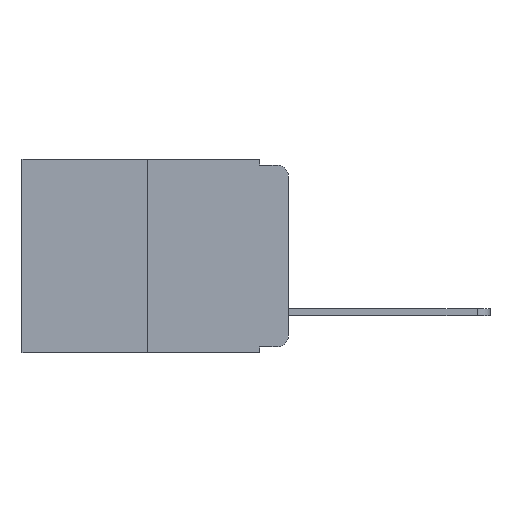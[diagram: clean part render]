
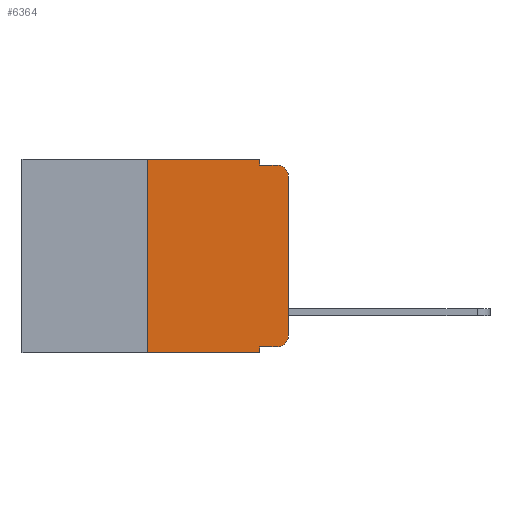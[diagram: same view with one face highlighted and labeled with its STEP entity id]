
A CAD part, left-side view. The second image highlights one B-rep face of the part: STEP entity #6364.
In plain terms, the highlighted planar face has unit normal (-1, 0, 0).
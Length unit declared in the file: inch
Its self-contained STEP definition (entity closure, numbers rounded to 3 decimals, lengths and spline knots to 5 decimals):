
#136 = CARTESIAN_POINT ( 'NONE',  ( 0., 0.02, -0.01 ) ) ;
#164 = CARTESIAN_POINT ( 'NONE',  ( 0., 0.051, 0. ) ) ;
#238 = EDGE_CURVE ( 'NONE', #1976, #2166, #1881, .T. ) ;
#375 = PLANE ( 'NONE',  #6137 ) ;
#435 = CARTESIAN_POINT ( 'NONE',  ( 0., 0.25, -0.343 ) ) ;
#563 = ORIENTED_EDGE ( 'NONE', *, *, #2200, .T. ) ;
#633 = VERTEX_POINT ( 'NONE', #4123 ) ;
#638 = FACE_OUTER_BOUND ( 'NONE', #3313, .T. ) ;
#803 = ORIENTED_EDGE ( 'NONE', *, *, #2149, .F. ) ;
#841 = VERTEX_POINT ( 'NONE', #3508 ) ;
#1305 = VERTEX_POINT ( 'NONE', #435 ) ;
#1477 = DIRECTION ( 'NONE',  ( 1., 0., 0. ) ) ;
#1661 = VECTOR ( 'NONE', #6414, 39.37008 ) ;
#1836 = CARTESIAN_POINT ( 'NONE',  ( 0., 0.02, -0.03 ) ) ;
#1881 = LINE ( 'NONE', #3683, #1661 ) ;
#1905 = EDGE_CURVE ( 'NONE', #1305, #4655, #7725, .T. ) ;
#1976 = VERTEX_POINT ( 'NONE', #6627 ) ;
#2124 = EDGE_CURVE ( 'NONE', #633, #841, #7049, .T. ) ;
#2126 = EDGE_CURVE ( 'NONE', #841, #3757, #6992, .T. ) ;
#2143 = EDGE_CURVE ( 'NONE', #8304, #3757, #7030, .T. ) ;
#2147 = EDGE_CURVE ( 'NONE', #2166, #8304, #6923, .T. ) ;
#2149 = EDGE_CURVE ( 'NONE', #1305, #1976, #6969, .T. ) ;
#2166 = VERTEX_POINT ( 'NONE', #2191 ) ;
#2179 = EDGE_CURVE ( 'NONE', #6156, #4655, #6856, .T. ) ;
#2191 = CARTESIAN_POINT ( 'NONE',  ( 0., 0.051, 0. ) ) ;
#2198 = EDGE_CURVE ( 'NONE', #6156, #2980, #6770, .T. ) ;
#2200 = EDGE_CURVE ( 'NONE', #2980, #633, #6793, .T. ) ;
#2881 = CARTESIAN_POINT ( 'NONE',  ( 0., 0.051, -0.01 ) ) ;
#2894 = DIRECTION ( 'NONE',  ( -1., 0., 0. ) ) ;
#2916 = DIRECTION ( 'NONE',  ( 0., 0., -1. ) ) ;
#2980 = VERTEX_POINT ( 'NONE', #4947 ) ;
#3180 = ORIENTED_EDGE ( 'NONE', *, *, #2124, .T. ) ;
#3198 = ORIENTED_EDGE ( 'NONE', *, *, #2143, .F. ) ;
#3262 = CARTESIAN_POINT ( 'NONE',  ( 0., 0.051, -0.333 ) ) ;
#3313 = EDGE_LOOP ( 'NONE', ( #3180, #3487, #3198, #3564, #3515, #803, #9243, #4069, #4049, #563 ) ) ;
#3487 = ORIENTED_EDGE ( 'NONE', *, *, #2126, .T. ) ;
#3508 = CARTESIAN_POINT ( 'NONE',  ( 0., 0., -0.03 ) ) ;
#3515 = ORIENTED_EDGE ( 'NONE', *, *, #238, .F. ) ;
#3564 = ORIENTED_EDGE ( 'NONE', *, *, #2147, .F. ) ;
#3683 = CARTESIAN_POINT ( 'NONE',  ( 0., 0.473, 0. ) ) ;
#3687 = DIRECTION ( 'NONE',  ( 0., 0., -1. ) ) ;
#3757 = VERTEX_POINT ( 'NONE', #136 ) ;
#4049 = ORIENTED_EDGE ( 'NONE', *, *, #2198, .T. ) ;
#4069 = ORIENTED_EDGE ( 'NONE', *, *, #2179, .F. ) ;
#4123 = CARTESIAN_POINT ( 'NONE',  ( 0., 0., -0.313 ) ) ;
#4212 = DIRECTION ( 'NONE',  ( 0., 0., -1. ) ) ;
#4518 = DIRECTION ( 'NONE',  ( 0., 0., 1. ) ) ;
#4655 = VERTEX_POINT ( 'NONE', #9818 ) ;
#4947 = CARTESIAN_POINT ( 'NONE',  ( 0., 0.02, -0.333 ) ) ;
#4954 = DIRECTION ( 'NONE',  ( 0., -1., 0. ) ) ;
#5167 = DIRECTION ( 'NONE',  ( 0., 0., -1. ) ) ;
#5472 = CARTESIAN_POINT ( 'NONE',  ( 0., 0.473, -0.343 ) ) ;
#5509 = CARTESIAN_POINT ( 'NONE',  ( 0., 0.051, 0. ) ) ;
#5519 = DIRECTION ( 'NONE',  ( 0., -1., 0. ) ) ;
#6137 = AXIS2_PLACEMENT_3D ( 'NONE', #7691, #1477, #7039 ) ;
#6156 = VERTEX_POINT ( 'NONE', #6898 ) ;
#6364 = ADVANCED_FACE ( 'NONE', ( #638 ), #375, .F. ) ;
#6414 = DIRECTION ( 'NONE',  ( 0., -1., 0. ) ) ;
#6627 = CARTESIAN_POINT ( 'NONE',  ( 0., 0.25, 0. ) ) ;
#6658 = DIRECTION ( 'NONE',  ( 0., -1., 0. ) ) ;
#6761 = VECTOR ( 'NONE', #4954, 39.37008 ) ;
#6770 = LINE ( 'NONE', #3262, #6761 ) ;
#6793 = CIRCLE ( 'NONE', #7742, 0.02 ) ;
#6821 = VECTOR ( 'NONE', #4212, 39.37008 ) ;
#6856 = LINE ( 'NONE', #5509, #6821 ) ;
#6890 = VECTOR ( 'NONE', #9769, 39.37008 ) ;
#6898 = CARTESIAN_POINT ( 'NONE',  ( 0., 0.051, -0.333 ) ) ;
#6905 = VECTOR ( 'NONE', #3687, 39.37008 ) ;
#6916 = VECTOR ( 'NONE', #5519, 39.37008 ) ;
#6923 = LINE ( 'NONE', #164, #6905 ) ;
#6969 = LINE ( 'NONE', #8595, #6890 ) ;
#6979 = VECTOR ( 'NONE', #4518, 39.37008 ) ;
#6992 = CIRCLE ( 'NONE', #7777, 0.02 ) ;
#7030 = LINE ( 'NONE', #7497, #6916 ) ;
#7039 = DIRECTION ( 'NONE',  ( 0., 0., -1. ) ) ;
#7049 = LINE ( 'NONE', #9753, #6979 ) ;
#7497 = CARTESIAN_POINT ( 'NONE',  ( 0., 0.051, -0.01 ) ) ;
#7691 = CARTESIAN_POINT ( 'NONE',  ( 0., 0.473, 0. ) ) ;
#7708 = VECTOR ( 'NONE', #6658, 39.37008 ) ;
#7725 = LINE ( 'NONE', #5472, #7708 ) ;
#7742 = AXIS2_PLACEMENT_3D ( 'NONE', #9786, #8008, #5167 ) ;
#7777 = AXIS2_PLACEMENT_3D ( 'NONE', #1836, #2894, #2916 ) ;
#8008 = DIRECTION ( 'NONE',  ( -1., 0., 0. ) ) ;
#8304 = VERTEX_POINT ( 'NONE', #2881 ) ;
#8595 = CARTESIAN_POINT ( 'NONE',  ( 0., 0.25, 0. ) ) ;
#9243 = ORIENTED_EDGE ( 'NONE', *, *, #1905, .T. ) ;
#9753 = CARTESIAN_POINT ( 'NONE',  ( 0., 0., 0. ) ) ;
#9769 = DIRECTION ( 'NONE',  ( 0., 0., 1. ) ) ;
#9786 = CARTESIAN_POINT ( 'NONE',  ( 0., 0.02, -0.313 ) ) ;
#9818 = CARTESIAN_POINT ( 'NONE',  ( 0., 0.051, -0.343 ) ) ;
